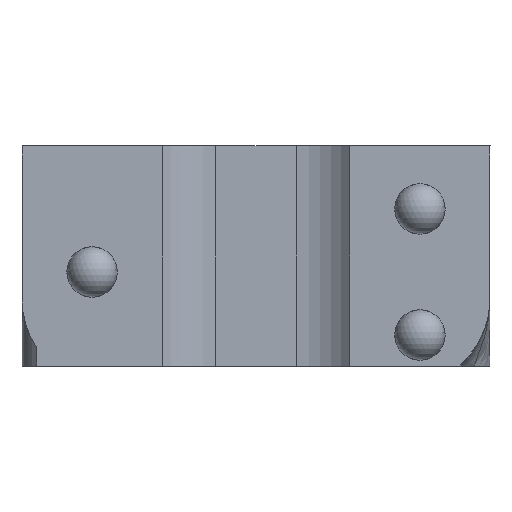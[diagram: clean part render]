
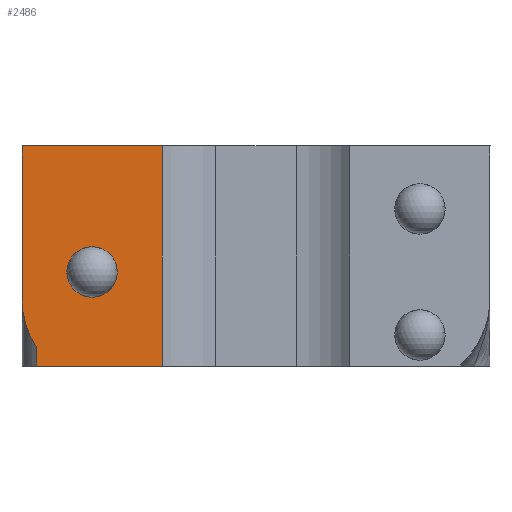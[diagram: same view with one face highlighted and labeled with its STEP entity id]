
A CAD part, left-side view. The second image highlights one B-rep face of the part: STEP entity #2486.
In plain terms, the highlighted planar face has unit normal (-1, 0, 0).
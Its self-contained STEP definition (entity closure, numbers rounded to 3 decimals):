
#95 = VERTEX_POINT ( 'NONE', #2079 ) ;
#143 = CARTESIAN_POINT ( 'NONE',  ( 82.199, 0.675, 3.815 ) ) ;
#253 = VERTEX_POINT ( 'NONE', #313 ) ;
#285 = DIRECTION ( 'NONE',  ( 0., 0., -1. ) ) ;
#313 = CARTESIAN_POINT ( 'NONE',  ( 82.199, 5.066, -3.647 ) ) ;
#330 = VERTEX_POINT ( 'NONE', #1798 ) ;
#357 = DIRECTION ( 'NONE',  ( -1., 0., 0. ) ) ;
#459 = EDGE_CURVE ( 'NONE', #1709, #95, #718, .T. ) ;
#461 = LINE ( 'NONE', #1547, #1693 ) ;
#529 = CARTESIAN_POINT ( 'NONE',  ( 82.199, 2.675, 3.815 ) ) ;
#588 = AXIS2_PLACEMENT_3D ( 'NONE', #143, #357, #2653 ) ;
#618 = EDGE_LOOP ( 'NONE', ( #1068, #2714, #1854, #3011, #2617, #1889 ) ) ;
#655 = DIRECTION ( 'NONE',  ( -1., 0., 0. ) ) ;
#675 = VECTOR ( 'NONE', #995, 1000. ) ;
#685 = VECTOR ( 'NONE', #2064, 1000. ) ;
#718 = LINE ( 'NONE', #2662, #1329 ) ;
#759 = CARTESIAN_POINT ( 'NONE',  ( 82.199, 6.232, 1.695 ) ) ;
#760 = CARTESIAN_POINT ( 'NONE',  ( 82.199, 5.066, -2.19 ) ) ;
#780 = DIRECTION ( 'NONE',  ( -1., 0., 0. ) ) ;
#805 = EDGE_LOOP ( 'NONE', ( #887, #1000 ) ) ;
#819 = CARTESIAN_POINT ( 'NONE',  ( 82.199, -4.883, -17.935 ) ) ;
#822 = EDGE_CURVE ( 'NONE', #1709, #330, #1966, .T. ) ;
#885 = EDGE_CURVE ( 'NONE', #2475, #1550, #1865, .T. ) ;
#887 = ORIENTED_EDGE ( 'NONE', *, *, #885, .F. ) ;
#995 = DIRECTION ( 'NONE',  ( 0., 0., -1. ) ) ;
#1000 = ORIENTED_EDGE ( 'NONE', *, *, #2864, .F. ) ;
#1057 = DIRECTION ( 'NONE',  ( 0., 1., 0. ) ) ;
#1068 = ORIENTED_EDGE ( 'NONE', *, *, #459, .T. ) ;
#1128 = CARTESIAN_POINT ( 'NONE',  ( 82.199, 69.175, 17.442 ) ) ;
#1142 = CARTESIAN_POINT ( 'NONE',  ( 82.199, 69.175, -3.647 ) ) ;
#1148 = EDGE_CURVE ( 'NONE', #2711, #95, #2537, .T. ) ;
#1166 = AXIS2_PLACEMENT_3D ( 'NONE', #1128, #2727, #1356 ) ;
#1206 = EDGE_CURVE ( 'NONE', #2476, #253, #461, .T. ) ;
#1300 = LINE ( 'NONE', #1142, #685 ) ;
#1329 = VECTOR ( 'NONE', #1057, 1000. ) ;
#1332 = FACE_OUTER_BOUND ( 'NONE', #618, .T. ) ;
#1356 = DIRECTION ( 'NONE',  ( 0., 1., 0. ) ) ;
#1413 = AXIS2_PLACEMENT_3D ( 'NONE', #2167, #780, #2407 ) ;
#1443 = CIRCLE ( 'NONE', #1552, 2. ) ;
#1547 = CARTESIAN_POINT ( 'NONE',  ( 82.199, 5.066, 7.452 ) ) ;
#1550 = VERTEX_POINT ( 'NONE', #2291 ) ;
#1552 = AXIS2_PLACEMENT_3D ( 'NONE', #2034, #655, #2271 ) ;
#1578 = VECTOR ( 'NONE', #2381, 1000. ) ;
#1693 = VECTOR ( 'NONE', #285, 1000. ) ;
#1709 = VERTEX_POINT ( 'NONE', #2637 ) ;
#1798 = CARTESIAN_POINT ( 'NONE',  ( 82.199, -4.883, -3.647 ) ) ;
#1854 = ORIENTED_EDGE ( 'NONE', *, *, #2819, .T. ) ;
#1865 = CIRCLE ( 'NONE', #588, 2. ) ;
#1889 = ORIENTED_EDGE ( 'NONE', *, *, #822, .F. ) ;
#1966 = LINE ( 'NONE', #819, #675 ) ;
#2034 = CARTESIAN_POINT ( 'NONE',  ( 82.199, 0.675, 3.815 ) ) ;
#2064 = DIRECTION ( 'NONE',  ( 0., -1., 0. ) ) ;
#2079 = CARTESIAN_POINT ( 'NONE',  ( 82.199, 6.232, 13.815 ) ) ;
#2167 = CARTESIAN_POINT ( 'NONE',  ( 82.199, -0.825, 1.695 ) ) ;
#2256 = EDGE_CURVE ( 'NONE', #253, #330, #1300, .T. ) ;
#2271 = DIRECTION ( 'NONE',  ( 0., 1., 0. ) ) ;
#2291 = CARTESIAN_POINT ( 'NONE',  ( 82.199, -1.325, 3.815 ) ) ;
#2381 = DIRECTION ( 'NONE',  ( 0., 0., 1. ) ) ;
#2407 = DIRECTION ( 'NONE',  ( 0., 1., 0. ) ) ;
#2420 = FACE_BOUND ( 'NONE', #805, .T. ) ;
#2475 = VERTEX_POINT ( 'NONE', #529 ) ;
#2476 = VERTEX_POINT ( 'NONE', #760 ) ;
#2486 = ADVANCED_FACE ( 'NONE', ( #1332, #2420 ), #2513, .F. ) ;
#2513 = PLANE ( 'NONE',  #1166 ) ;
#2537 = LINE ( 'NONE', #759, #1578 ) ;
#2617 = ORIENTED_EDGE ( 'NONE', *, *, #2256, .T. ) ;
#2637 = CARTESIAN_POINT ( 'NONE',  ( 82.199, -4.883, 13.815 ) ) ;
#2653 = DIRECTION ( 'NONE',  ( 0., 1., 0. ) ) ;
#2662 = CARTESIAN_POINT ( 'NONE',  ( 82.199, 1.953, 13.815 ) ) ;
#2711 = VERTEX_POINT ( 'NONE', #2808 ) ;
#2714 = ORIENTED_EDGE ( 'NONE', *, *, #1148, .F. ) ;
#2727 = DIRECTION ( 'NONE',  ( 1., 0., 0. ) ) ;
#2808 = CARTESIAN_POINT ( 'NONE',  ( 82.199, 6.232, 1.695 ) ) ;
#2819 = EDGE_CURVE ( 'NONE', #2711, #2476, #2876, .T. ) ;
#2864 = EDGE_CURVE ( 'NONE', #1550, #2475, #1443, .T. ) ;
#2876 = CIRCLE ( 'NONE', #1413, 7.057 ) ;
#3011 = ORIENTED_EDGE ( 'NONE', *, *, #1206, .T. ) ;
